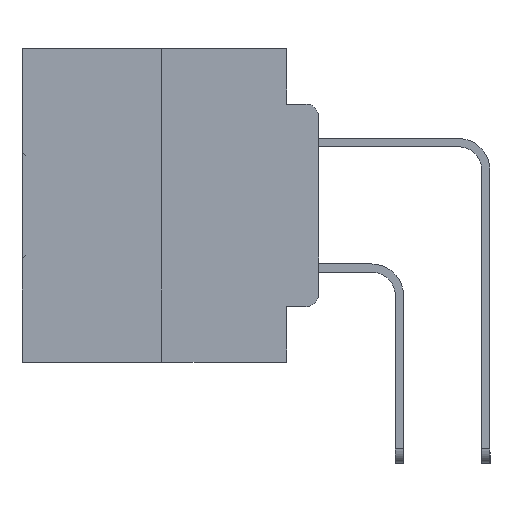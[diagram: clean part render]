
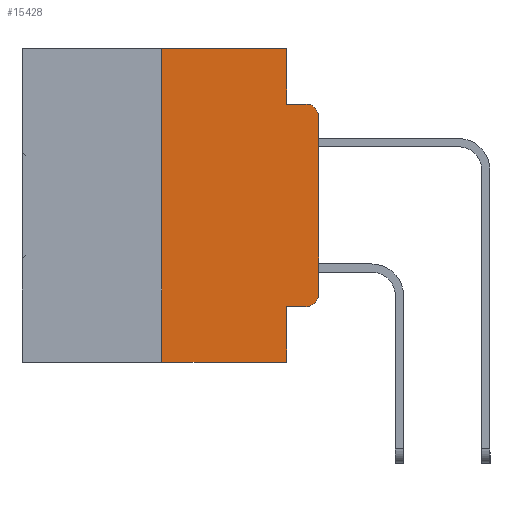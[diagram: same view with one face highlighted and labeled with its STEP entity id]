
A CAD part, left-side view. The second image highlights one B-rep face of the part: STEP entity #15428.
In plain terms, the highlighted planar face has unit normal (-1, 0, 0).
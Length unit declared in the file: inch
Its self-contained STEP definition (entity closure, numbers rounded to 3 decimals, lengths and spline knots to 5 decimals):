
#1135 = CARTESIAN_POINT ( 'NONE',  ( 0., 0.25, 0. ) ) ;
#1839 = VERTEX_POINT ( 'NONE', #5759 ) ;
#2486 = LINE ( 'NONE', #20696, #23381 ) ;
#2835 = ORIENTED_EDGE ( 'NONE', *, *, #5218, .T. ) ;
#3664 = AXIS2_PLACEMENT_3D ( 'NONE', #26249, #10514, #28838 ) ;
#4167 = CARTESIAN_POINT ( 'NONE',  ( 0., 0.473, 0. ) ) ;
#4683 = FACE_OUTER_BOUND ( 'NONE', #11868, .T. ) ;
#4963 = CARTESIAN_POINT ( 'NONE',  ( 0., 0.25, 0. ) ) ;
#5148 = EDGE_CURVE ( 'NONE', #1839, #29239, #12763, .T. ) ;
#5218 = EDGE_CURVE ( 'NONE', #24425, #17820, #22627, .T. ) ;
#5364 = DIRECTION ( 'NONE',  ( 0., -1., 0. ) ) ;
#5390 = CARTESIAN_POINT ( 'NONE',  ( 0., 0., 0. ) ) ;
#5570 = DIRECTION ( 'NONE',  ( 0., 0., -1. ) ) ;
#5759 = CARTESIAN_POINT ( 'NONE',  ( 0., 0.25, -0.5 ) ) ;
#6621 = EDGE_CURVE ( 'NONE', #25322, #24425, #13419, .T. ) ;
#6754 = DIRECTION ( 'NONE',  ( 1., 0., 0. ) ) ;
#6914 = VERTEX_POINT ( 'NONE', #14537 ) ;
#7056 = CARTESIAN_POINT ( 'NONE',  ( 0., 0.051, -0.0885 ) ) ;
#7382 = LINE ( 'NONE', #7056, #21343 ) ;
#7460 = DIRECTION ( 'NONE',  ( 0., -1., 0. ) ) ;
#7617 = DIRECTION ( 'NONE',  ( 0., -1., 0. ) ) ;
#7709 = LINE ( 'NONE', #25506, #16338 ) ;
#8036 = ORIENTED_EDGE ( 'NONE', *, *, #21688, .T. ) ;
#8282 = EDGE_CURVE ( 'NONE', #26000, #25322, #25189, .T. ) ;
#8426 = ORIENTED_EDGE ( 'NONE', *, *, #8282, .T. ) ;
#10514 = DIRECTION ( 'NONE',  ( -1., 0., 0. ) ) ;
#11085 = VECTOR ( 'NONE', #7460, 39.37008 ) ;
#11566 = EDGE_CURVE ( 'NONE', #14586, #28650, #25848, .T. ) ;
#11614 = EDGE_CURVE ( 'NONE', #23104, #29239, #31084, .T. ) ;
#11868 = EDGE_LOOP ( 'NONE', ( #15017, #2835, #14123, #25576, #29595, #17468, #26109, #13376, #8036, #8426 ) ) ;
#12573 = VECTOR ( 'NONE', #21088, 39.37008 ) ;
#12763 = LINE ( 'NONE', #25809, #11085 ) ;
#12904 = AXIS2_PLACEMENT_3D ( 'NONE', #30411, #14794, #32967 ) ;
#13061 = CARTESIAN_POINT ( 'NONE',  ( 0., 0., -0.1085 ) ) ;
#13362 = CARTESIAN_POINT ( 'NONE',  ( 0., 0.051, 0. ) ) ;
#13376 = ORIENTED_EDGE ( 'NONE', *, *, #11614, .F. ) ;
#13419 = LINE ( 'NONE', #5390, #12573 ) ;
#13962 = CARTESIAN_POINT ( 'NONE',  ( 0., 0.02, -0.0885 ) ) ;
#14123 = ORIENTED_EDGE ( 'NONE', *, *, #21567, .F. ) ;
#14195 = DIRECTION ( 'NONE',  ( 0., 0., 1. ) ) ;
#14537 = CARTESIAN_POINT ( 'NONE',  ( 0., 0.051, -0.0885 ) ) ;
#14586 = VERTEX_POINT ( 'NONE', #4963 ) ;
#14794 = DIRECTION ( 'NONE',  ( -1., 0., 0. ) ) ;
#15017 = ORIENTED_EDGE ( 'NONE', *, *, #6621, .T. ) ;
#15428 = ADVANCED_FACE ( 'NONE', ( #4683 ), #19821, .F. ) ;
#16338 = VECTOR ( 'NONE', #27999, 39.37008 ) ;
#16458 = VECTOR ( 'NONE', #14195, 39.37008 ) ;
#17206 = VECTOR ( 'NONE', #5570, 39.37008 ) ;
#17468 = ORIENTED_EDGE ( 'NONE', *, *, #21359, .F. ) ;
#17820 = VERTEX_POINT ( 'NONE', #13962 ) ;
#18852 = VECTOR ( 'NONE', #5364, 39.37008 ) ;
#19821 = PLANE ( 'NONE',  #31643 ) ;
#20003 = DIRECTION ( 'NONE',  ( 0., -1., 0. ) ) ;
#20696 = CARTESIAN_POINT ( 'NONE',  ( 0., 0.051, -0.4115 ) ) ;
#21088 = DIRECTION ( 'NONE',  ( 0., 0., 1. ) ) ;
#21343 = VECTOR ( 'NONE', #20003, 39.37008 ) ;
#21359 = EDGE_CURVE ( 'NONE', #1839, #14586, #23446, .T. ) ;
#21567 = EDGE_CURVE ( 'NONE', #6914, #17820, #7382, .T. ) ;
#21688 = EDGE_CURVE ( 'NONE', #23104, #26000, #2486, .T. ) ;
#22385 = CARTESIAN_POINT ( 'NONE',  ( 0., 0.02, -0.4115 ) ) ;
#22627 = CIRCLE ( 'NONE', #3664, 0.02 ) ;
#23104 = VERTEX_POINT ( 'NONE', #29372 ) ;
#23381 = VECTOR ( 'NONE', #7617, 39.37008 ) ;
#23446 = LINE ( 'NONE', #1135, #16458 ) ;
#24425 = VERTEX_POINT ( 'NONE', #13061 ) ;
#24583 = CARTESIAN_POINT ( 'NONE',  ( 0., 0., -0.3915 ) ) ;
#25097 = DIRECTION ( 'NONE',  ( 0., 0., -1. ) ) ;
#25189 = CIRCLE ( 'NONE', #12904, 0.02 ) ;
#25322 = VERTEX_POINT ( 'NONE', #24583 ) ;
#25506 = CARTESIAN_POINT ( 'NONE',  ( 0., 0.051, 0. ) ) ;
#25576 = ORIENTED_EDGE ( 'NONE', *, *, #32264, .F. ) ;
#25809 = CARTESIAN_POINT ( 'NONE',  ( 0., 0.473, -0.5 ) ) ;
#25848 = LINE ( 'NONE', #26316, #18852 ) ;
#26000 = VERTEX_POINT ( 'NONE', #22385 ) ;
#26109 = ORIENTED_EDGE ( 'NONE', *, *, #5148, .T. ) ;
#26249 = CARTESIAN_POINT ( 'NONE',  ( 0., 0.02, -0.1085 ) ) ;
#26316 = CARTESIAN_POINT ( 'NONE',  ( 0., 0.473, 0. ) ) ;
#27999 = DIRECTION ( 'NONE',  ( 0., 0., -1. ) ) ;
#28650 = VERTEX_POINT ( 'NONE', #29677 ) ;
#28838 = DIRECTION ( 'NONE',  ( 0., 0., -1. ) ) ;
#29239 = VERTEX_POINT ( 'NONE', #31996 ) ;
#29372 = CARTESIAN_POINT ( 'NONE',  ( 0., 0.051, -0.4115 ) ) ;
#29595 = ORIENTED_EDGE ( 'NONE', *, *, #11566, .F. ) ;
#29677 = CARTESIAN_POINT ( 'NONE',  ( 0., 0.051, 0. ) ) ;
#30411 = CARTESIAN_POINT ( 'NONE',  ( 0., 0.02, -0.3915 ) ) ;
#31084 = LINE ( 'NONE', #13362, #17206 ) ;
#31643 = AXIS2_PLACEMENT_3D ( 'NONE', #4167, #6754, #25097 ) ;
#31996 = CARTESIAN_POINT ( 'NONE',  ( 0., 0.051, -0.5 ) ) ;
#32264 = EDGE_CURVE ( 'NONE', #28650, #6914, #7709, .T. ) ;
#32967 = DIRECTION ( 'NONE',  ( 0., 0., -1. ) ) ;
